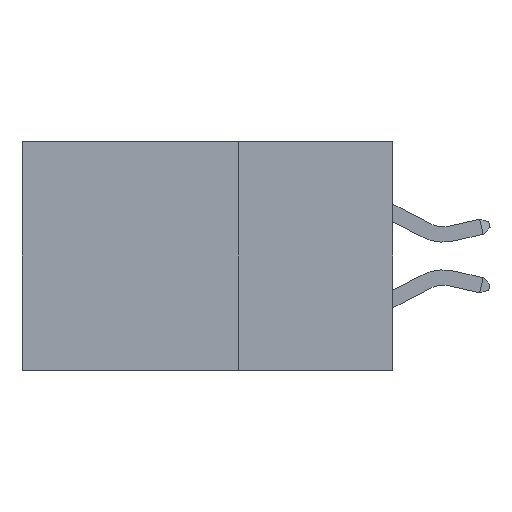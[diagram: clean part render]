
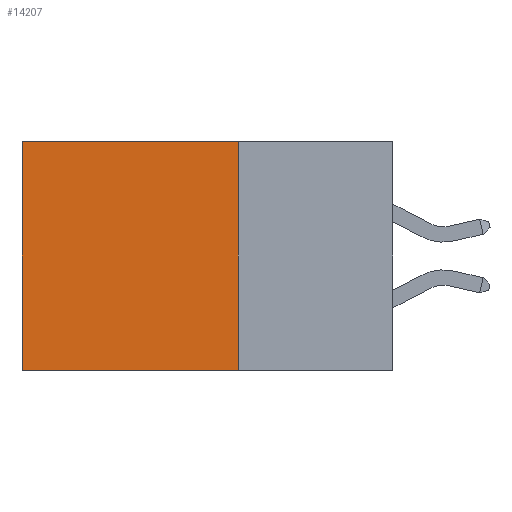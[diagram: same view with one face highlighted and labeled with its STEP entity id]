
A CAD part, left-side view. The second image highlights one B-rep face of the part: STEP entity #14207.
In plain terms, the highlighted planar face has unit normal (-1, 0, 0).
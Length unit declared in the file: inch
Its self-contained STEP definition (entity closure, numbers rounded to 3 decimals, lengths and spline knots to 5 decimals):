
#325 = LINE ( 'NONE', #27958, #17594 ) ;
#994 = VECTOR ( 'NONE', #23872, 39.37008 ) ;
#2126 = PLANE ( 'NONE',  #24739 ) ;
#2288 = CARTESIAN_POINT ( 'NONE',  ( 0.2875, 0.6, -0.37 ) ) ;
#2319 = CARTESIAN_POINT ( 'NONE',  ( 0.2875, 0.25, 0. ) ) ;
#2679 = ORIENTED_EDGE ( 'NONE', *, *, #11477, .T. ) ;
#2861 = FACE_OUTER_BOUND ( 'NONE', #21185, .T. ) ;
#3277 = VERTEX_POINT ( 'NONE', #2288 ) ;
#6730 = LINE ( 'NONE', #8553, #994 ) ;
#7256 = VECTOR ( 'NONE', #23656, 39.37008 ) ;
#7466 = LINE ( 'NONE', #24054, #22390 ) ;
#8420 = EDGE_CURVE ( 'NONE', #11418, #14273, #325, .T. ) ;
#8553 = CARTESIAN_POINT ( 'NONE',  ( 0.2875, 0.6, 0. ) ) ;
#9318 = LINE ( 'NONE', #17139, #7256 ) ;
#10345 = EDGE_CURVE ( 'NONE', #14363, #3277, #7466, .T. ) ;
#11102 = DIRECTION ( 'NONE',  ( 1., 0., 0. ) ) ;
#11418 = VERTEX_POINT ( 'NONE', #21127 ) ;
#11477 = EDGE_CURVE ( 'NONE', #14273, #3277, #6730, .T. ) ;
#14207 = ADVANCED_FACE ( 'NONE', ( #2861 ), #2126, .F. ) ;
#14273 = VERTEX_POINT ( 'NONE', #21460 ) ;
#14363 = VERTEX_POINT ( 'NONE', #21821 ) ;
#17139 = CARTESIAN_POINT ( 'NONE',  ( 0.2875, 0.25, 0. ) ) ;
#17258 = DIRECTION ( 'NONE',  ( 0., 1., 0. ) ) ;
#17444 = DIRECTION ( 'NONE',  ( 0., 0., -1. ) ) ;
#17594 = VECTOR ( 'NONE', #25404, 39.37008 ) ;
#21025 = ORIENTED_EDGE ( 'NONE', *, *, #10345, .F. ) ;
#21127 = CARTESIAN_POINT ( 'NONE',  ( 0.2875, 0.25, 0. ) ) ;
#21185 = EDGE_LOOP ( 'NONE', ( #2679, #21025, #21859, #22881 ) ) ;
#21460 = CARTESIAN_POINT ( 'NONE',  ( 0.2875, 0.6, 0. ) ) ;
#21821 = CARTESIAN_POINT ( 'NONE',  ( 0.2875, 0.25, -0.37 ) ) ;
#21859 = ORIENTED_EDGE ( 'NONE', *, *, #23408, .F. ) ;
#22390 = VECTOR ( 'NONE', #17258, 39.37008 ) ;
#22881 = ORIENTED_EDGE ( 'NONE', *, *, #8420, .T. ) ;
#23408 = EDGE_CURVE ( 'NONE', #11418, #14363, #9318, .T. ) ;
#23656 = DIRECTION ( 'NONE',  ( 0., 0., -1. ) ) ;
#23872 = DIRECTION ( 'NONE',  ( 0., 0., -1. ) ) ;
#24054 = CARTESIAN_POINT ( 'NONE',  ( 0.2875, 0.25, -0.37 ) ) ;
#24739 = AXIS2_PLACEMENT_3D ( 'NONE', #2319, #11102, #17444 ) ;
#25404 = DIRECTION ( 'NONE',  ( 0., 1., 0. ) ) ;
#27958 = CARTESIAN_POINT ( 'NONE',  ( 0.2875, 0.25, 0. ) ) ;
